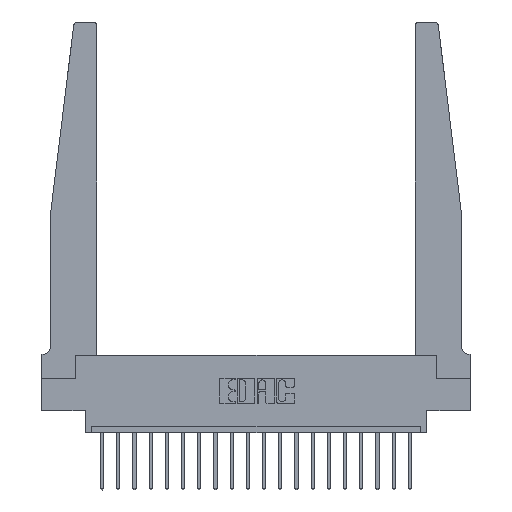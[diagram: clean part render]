
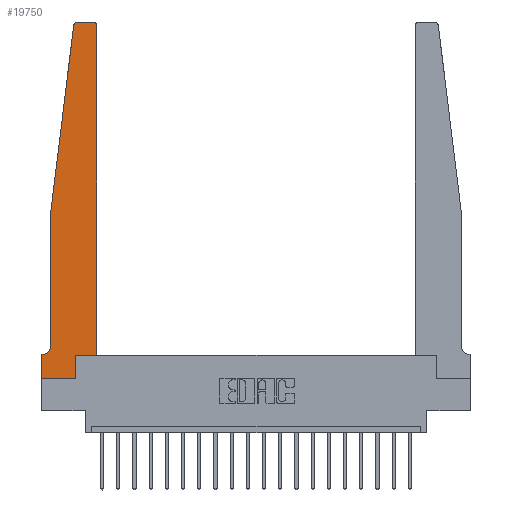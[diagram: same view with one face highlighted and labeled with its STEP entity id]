
A CAD part, top view. The second image highlights one B-rep face of the part: STEP entity #19750.
In plain terms, the highlighted planar face has unit normal (0, 0, 1).
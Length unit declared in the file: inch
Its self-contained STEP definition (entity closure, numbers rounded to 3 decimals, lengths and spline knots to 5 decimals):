
#76 = CARTESIAN_POINT ( 'NONE',  ( 0.015, 0.2375, 0.37 ) ) ;
#132 = LINE ( 'NONE', #15969, #18013 ) ;
#369 = LINE ( 'NONE', #14518, #7214 ) ;
#514 = ORIENTED_EDGE ( 'NONE', *, *, #18137, .T. ) ;
#794 = VERTEX_POINT ( 'NONE', #13755 ) ;
#926 = DIRECTION ( 'NONE',  ( 0., -1., 0. ) ) ;
#1206 = DIRECTION ( 'NONE',  ( 0., 0., 1. ) ) ;
#1219 = ORIENTED_EDGE ( 'NONE', *, *, #10988, .T. ) ;
#1408 = VERTEX_POINT ( 'NONE', #17367 ) ;
#1474 = VERTEX_POINT ( 'NONE', #9602 ) ;
#1559 = CARTESIAN_POINT ( 'NONE',  ( 0.2605, 0.18, 0.37 ) ) ;
#1619 = ORIENTED_EDGE ( 'NONE', *, *, #7013, .T. ) ;
#1735 = VECTOR ( 'NONE', #1921, 39.37008 ) ;
#1921 = DIRECTION ( 'NONE',  ( -1., 0., 0. ) ) ;
#1933 = EDGE_CURVE ( 'NONE', #12445, #7662, #2898, .T. ) ;
#2013 = DIRECTION ( 'NONE',  ( 1., 0., 0. ) ) ;
#2122 = LINE ( 'NONE', #1559, #18297 ) ;
#2281 = CARTESIAN_POINT ( 'NONE',  ( 0.065, 1.25, 0.37 ) ) ;
#2330 = ORIENTED_EDGE ( 'NONE', *, *, #16495, .T. ) ;
#2412 = DIRECTION ( 'NONE',  ( -0.122, -0.992, 0. ) ) ;
#2633 = ORIENTED_EDGE ( 'NONE', *, *, #4831, .T. ) ;
#2898 = LINE ( 'NONE', #17904, #18105 ) ;
#3188 = LINE ( 'NONE', #19320, #1735 ) ;
#3220 = CARTESIAN_POINT ( 'NONE',  ( 0.065, 0.1875, 0.37 ) ) ;
#3258 = VERTEX_POINT ( 'NONE', #11651 ) ;
#4001 = CARTESIAN_POINT ( 'NONE',  ( 0.015, 0.1875, 0.37 ) ) ;
#4831 = EDGE_CURVE ( 'NONE', #6482, #794, #17019, .T. ) ;
#5245 = EDGE_CURVE ( 'NONE', #15441, #12445, #17479, .T. ) ;
#5360 = ORIENTED_EDGE ( 'NONE', *, *, #7586, .T. ) ;
#5622 = AXIS2_PLACEMENT_3D ( 'NONE', #16573, #14897, #18086 ) ;
#5847 = LINE ( 'NONE', #2281, #15888 ) ;
#6234 = CIRCLE ( 'NONE', #8819, 0.05 ) ;
#6482 = VERTEX_POINT ( 'NONE', #10418 ) ;
#6733 = ORIENTED_EDGE ( 'NONE', *, *, #10155, .T. ) ;
#6800 = AXIS2_PLACEMENT_3D ( 'NONE', #10601, #13524, #8872 ) ;
#7013 = EDGE_CURVE ( 'NONE', #11564, #1474, #11235, .T. ) ;
#7214 = VECTOR ( 'NONE', #2013, 39.37008 ) ;
#7586 = EDGE_CURVE ( 'NONE', #3258, #11564, #11071, .T. ) ;
#7662 = VERTEX_POINT ( 'NONE', #17395 ) ;
#8113 = CARTESIAN_POINT ( 'NONE',  ( 0.2605, 0.18, 0.37 ) ) ;
#8819 = AXIS2_PLACEMENT_3D ( 'NONE', #76, #14183, #12606 ) ;
#8872 = DIRECTION ( 'NONE',  ( 1., 0., 0. ) ) ;
#9119 = VECTOR ( 'NONE', #20290, 39.37008 ) ;
#9602 = CARTESIAN_POINT ( 'NONE',  ( 0.395, 2.75, 0.37 ) ) ;
#9766 = ORIENTED_EDGE ( 'NONE', *, *, #15171, .T. ) ;
#10155 = EDGE_CURVE ( 'NONE', #11985, #1408, #16381, .T. ) ;
#10418 = CARTESIAN_POINT ( 'NONE',  ( 0.065, 1.25, 0.37 ) ) ;
#10601 = CARTESIAN_POINT ( 'NONE',  ( 0., 0.1875, 0.37 ) ) ;
#10913 = CARTESIAN_POINT ( 'NONE',  ( 0.425, 2.72, 0.37 ) ) ;
#10988 = EDGE_CURVE ( 'NONE', #15336, #19308, #2122, .T. ) ;
#11071 = LINE ( 'NONE', #18638, #15476 ) ;
#11235 = CIRCLE ( 'NONE', #20063, 0.03 ) ;
#11564 = VERTEX_POINT ( 'NONE', #10913 ) ;
#11593 = CARTESIAN_POINT ( 'NONE',  ( 0.065, 1.25, 0.37 ) ) ;
#11651 = CARTESIAN_POINT ( 'NONE',  ( 0.425, 0.18, 0.37 ) ) ;
#11985 = VERTEX_POINT ( 'NONE', #16670 ) ;
#12445 = VERTEX_POINT ( 'NONE', #13830 ) ;
#12606 = DIRECTION ( 'NONE',  ( -1., 0., 0. ) ) ;
#13052 = EDGE_CURVE ( 'NONE', #794, #15441, #6234, .T. ) ;
#13524 = DIRECTION ( 'NONE',  ( 0., 0., 1. ) ) ;
#13755 = CARTESIAN_POINT ( 'NONE',  ( 0.065, 0.2375, 0.37 ) ) ;
#13830 = CARTESIAN_POINT ( 'NONE',  ( 0., 0.1875, 0.37 ) ) ;
#13872 = ORIENTED_EDGE ( 'NONE', *, *, #18772, .T. ) ;
#14183 = DIRECTION ( 'NONE',  ( 0., 0., -1. ) ) ;
#14321 = CARTESIAN_POINT ( 'NONE',  ( 0.2605, 0., 0.37 ) ) ;
#14518 = CARTESIAN_POINT ( 'NONE',  ( 0., 0., 0.37 ) ) ;
#14728 = ORIENTED_EDGE ( 'NONE', *, *, #5245, .T. ) ;
#14897 = DIRECTION ( 'NONE',  ( 0., 0., 1. ) ) ;
#15171 = EDGE_CURVE ( 'NONE', #1474, #11985, #3188, .T. ) ;
#15336 = VERTEX_POINT ( 'NONE', #14321 ) ;
#15436 = DIRECTION ( 'NONE',  ( 1., 0., 0. ) ) ;
#15441 = VERTEX_POINT ( 'NONE', #4001 ) ;
#15476 = VECTOR ( 'NONE', #15602, 39.37008 ) ;
#15602 = DIRECTION ( 'NONE',  ( 0., 1., 0. ) ) ;
#15888 = VECTOR ( 'NONE', #2412, 39.37008 ) ;
#15969 = CARTESIAN_POINT ( 'NONE',  ( 0.425, 0.18, 0.37 ) ) ;
#16131 = EDGE_LOOP ( 'NONE', ( #9766, #6733, #2330, #2633, #16451, #14728, #19833, #514, #1219, #13872, #5360, #1619 ) ) ;
#16181 = DIRECTION ( 'NONE',  ( 0., 1., 0. ) ) ;
#16381 = CIRCLE ( 'NONE', #5622, 0.03 ) ;
#16451 = ORIENTED_EDGE ( 'NONE', *, *, #13052, .T. ) ;
#16495 = EDGE_CURVE ( 'NONE', #1408, #6482, #5847, .T. ) ;
#16573 = CARTESIAN_POINT ( 'NONE',  ( 0.27653, 2.72, 0.37 ) ) ;
#16670 = CARTESIAN_POINT ( 'NONE',  ( 0.27653, 2.75, 0.37 ) ) ;
#16744 = VECTOR ( 'NONE', #926, 39.37008 ) ;
#17019 = LINE ( 'NONE', #11593, #16744 ) ;
#17367 = CARTESIAN_POINT ( 'NONE',  ( 0.24675, 2.72367, 0.37 ) ) ;
#17395 = CARTESIAN_POINT ( 'NONE',  ( 0., 0., 0.37 ) ) ;
#17479 = LINE ( 'NONE', #3220, #9119 ) ;
#17683 = DIRECTION ( 'NONE',  ( 1., 0., 0. ) ) ;
#17762 = FACE_OUTER_BOUND ( 'NONE', #16131, .T. ) ;
#17904 = CARTESIAN_POINT ( 'NONE',  ( 0., 0., 0.37 ) ) ;
#18013 = VECTOR ( 'NONE', #17683, 39.37008 ) ;
#18086 = DIRECTION ( 'NONE',  ( 1., 0., 0. ) ) ;
#18105 = VECTOR ( 'NONE', #19414, 39.37008 ) ;
#18137 = EDGE_CURVE ( 'NONE', #7662, #15336, #369, .T. ) ;
#18297 = VECTOR ( 'NONE', #16181, 39.37008 ) ;
#18638 = CARTESIAN_POINT ( 'NONE',  ( 0.425, 0.18, 0.37 ) ) ;
#18772 = EDGE_CURVE ( 'NONE', #19308, #3258, #132, .T. ) ;
#19308 = VERTEX_POINT ( 'NONE', #8113 ) ;
#19320 = CARTESIAN_POINT ( 'NONE',  ( 0.25, 2.75, 0.37 ) ) ;
#19414 = DIRECTION ( 'NONE',  ( 0., -1., 0. ) ) ;
#19750 = ADVANCED_FACE ( 'NONE', ( #17762 ), #19778, .T. ) ;
#19778 = PLANE ( 'NONE',  #6800 ) ;
#19833 = ORIENTED_EDGE ( 'NONE', *, *, #1933, .T. ) ;
#20050 = CARTESIAN_POINT ( 'NONE',  ( 0.395, 2.72, 0.37 ) ) ;
#20063 = AXIS2_PLACEMENT_3D ( 'NONE', #20050, #1206, #15436 ) ;
#20290 = DIRECTION ( 'NONE',  ( -1., 0., 0. ) ) ;
